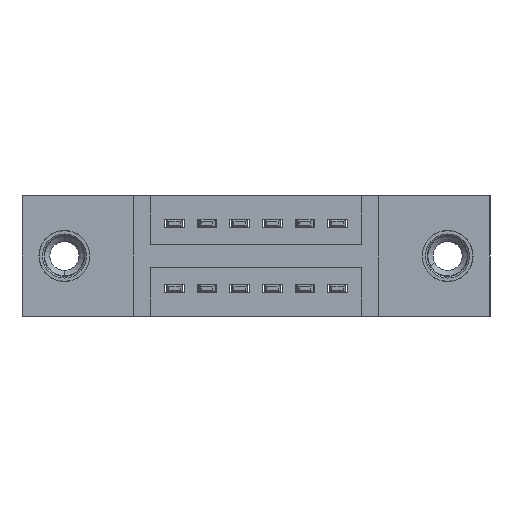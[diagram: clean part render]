
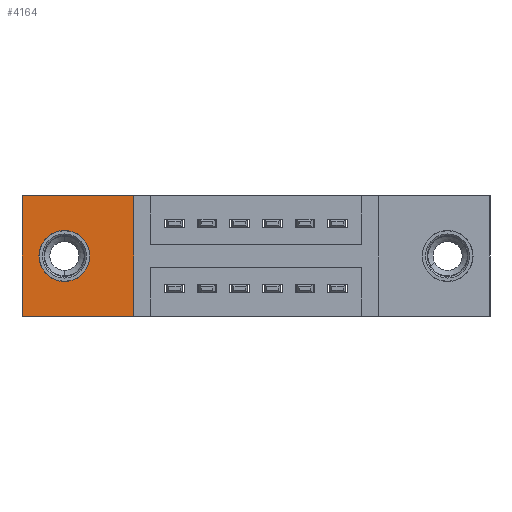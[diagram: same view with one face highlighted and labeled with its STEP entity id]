
A CAD part, front view. The second image highlights one B-rep face of the part: STEP entity #4164.
In plain terms, the highlighted planar face has unit normal (0, -1, 0).
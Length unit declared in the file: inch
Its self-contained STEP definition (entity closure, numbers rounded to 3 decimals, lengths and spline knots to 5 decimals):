
#4 = LINE ( 'NONE', #2674, #4541 ) ;
#246 = ORIENTED_EDGE ( 'NONE', *, *, #1412, .T. ) ;
#279 = VECTOR ( 'NONE', #10102, 39.37008 ) ;
#303 = VERTEX_POINT ( 'NONE', #4742 ) ;
#330 = ORIENTED_EDGE ( 'NONE', *, *, #6564, .F. ) ;
#437 = EDGE_LOOP ( 'NONE', ( #246, #9528, #9617, #9332 ) ) ;
#467 = VERTEX_POINT ( 'NONE', #6284 ) ;
#661 = LINE ( 'NONE', #5459, #8022 ) ;
#702 = FACE_BOUND ( 'NONE', #7304, .T. ) ;
#751 = AXIS2_PLACEMENT_3D ( 'NONE', #8159, #7402, #7446 ) ;
#991 = CARTESIAN_POINT ( 'NONE',  ( 0.3425, 0.17, 0. ) ) ;
#1412 = EDGE_CURVE ( 'NONE', #303, #467, #7996, .T. ) ;
#1536 = EDGE_CURVE ( 'NONE', #10074, #6081, #7205, .T. ) ;
#1884 = CARTESIAN_POINT ( 'NONE',  ( 0., 0.17, -0.37 ) ) ;
#2674 = CARTESIAN_POINT ( 'NONE',  ( 0., 0.17, -0.37 ) ) ;
#3086 = CIRCLE ( 'NONE', #751, 0.078 ) ;
#3400 = CARTESIAN_POINT ( 'NONE',  ( 0.13, 0.17, -0.185 ) ) ;
#3401 = DIRECTION ( 'NONE',  ( 1., 0., 0. ) ) ;
#3438 = DIRECTION ( 'NONE',  ( 0., 0., -1. ) ) ;
#3476 = CARTESIAN_POINT ( 'NONE',  ( 0.13, 0.17, -0.107 ) ) ;
#4058 = CARTESIAN_POINT ( 'NONE',  ( 0.3425, 0.17, -0.37 ) ) ;
#4164 = ADVANCED_FACE ( 'NONE', ( #702, #9223 ), #6704, .T. ) ;
#4457 = CARTESIAN_POINT ( 'NONE',  ( 0.3425, 0.17, 0. ) ) ;
#4541 = VECTOR ( 'NONE', #3401, 39.37008 ) ;
#4605 = DIRECTION ( 'NONE',  ( -1., 0., 0. ) ) ;
#4742 = CARTESIAN_POINT ( 'NONE',  ( 0., 0.17, 0. ) ) ;
#4764 = CARTESIAN_POINT ( 'NONE',  ( 0.13, 0.17, -0.263 ) ) ;
#4919 = VERTEX_POINT ( 'NONE', #3476 ) ;
#5133 = DIRECTION ( 'NONE',  ( 0., 0., -1. ) ) ;
#5250 = VERTEX_POINT ( 'NONE', #4764 ) ;
#5459 = CARTESIAN_POINT ( 'NONE',  ( 0., 0.17, 0. ) ) ;
#6081 = VERTEX_POINT ( 'NONE', #4457 ) ;
#6176 = EDGE_CURVE ( 'NONE', #6081, #303, #661, .T. ) ;
#6284 = CARTESIAN_POINT ( 'NONE',  ( 0., 0.17, -0.37 ) ) ;
#6564 = EDGE_CURVE ( 'NONE', #4919, #5250, #7901, .T. ) ;
#6704 = PLANE ( 'NONE',  #9629 ) ;
#7057 = EDGE_CURVE ( 'NONE', #467, #10074, #4, .T. ) ;
#7205 = LINE ( 'NONE', #991, #279 ) ;
#7270 = AXIS2_PLACEMENT_3D ( 'NONE', #3400, #8450, #3438 ) ;
#7304 = EDGE_LOOP ( 'NONE', ( #330, #8462 ) ) ;
#7402 = DIRECTION ( 'NONE',  ( 0., -1., 0. ) ) ;
#7446 = DIRECTION ( 'NONE',  ( 0., 0., -1. ) ) ;
#7901 = CIRCLE ( 'NONE', #7270, 0.078 ) ;
#7996 = LINE ( 'NONE', #10587, #10459 ) ;
#8022 = VECTOR ( 'NONE', #4605, 39.37008 ) ;
#8159 = CARTESIAN_POINT ( 'NONE',  ( 0.13, 0.17, -0.185 ) ) ;
#8402 = DIRECTION ( 'NONE',  ( 0., -1., 0. ) ) ;
#8450 = DIRECTION ( 'NONE',  ( 0., -1., 0. ) ) ;
#8462 = ORIENTED_EDGE ( 'NONE', *, *, #8924, .F. ) ;
#8924 = EDGE_CURVE ( 'NONE', #5250, #4919, #3086, .T. ) ;
#8953 = DIRECTION ( 'NONE',  ( 0., 0., -1. ) ) ;
#9223 = FACE_OUTER_BOUND ( 'NONE', #437, .T. ) ;
#9332 = ORIENTED_EDGE ( 'NONE', *, *, #6176, .T. ) ;
#9528 = ORIENTED_EDGE ( 'NONE', *, *, #7057, .T. ) ;
#9617 = ORIENTED_EDGE ( 'NONE', *, *, #1536, .T. ) ;
#9629 = AXIS2_PLACEMENT_3D ( 'NONE', #1884, #8402, #5133 ) ;
#10074 = VERTEX_POINT ( 'NONE', #4058 ) ;
#10102 = DIRECTION ( 'NONE',  ( 0., 0., 1. ) ) ;
#10459 = VECTOR ( 'NONE', #8953, 39.37008 ) ;
#10587 = CARTESIAN_POINT ( 'NONE',  ( 0., 0.17, 0. ) ) ;
